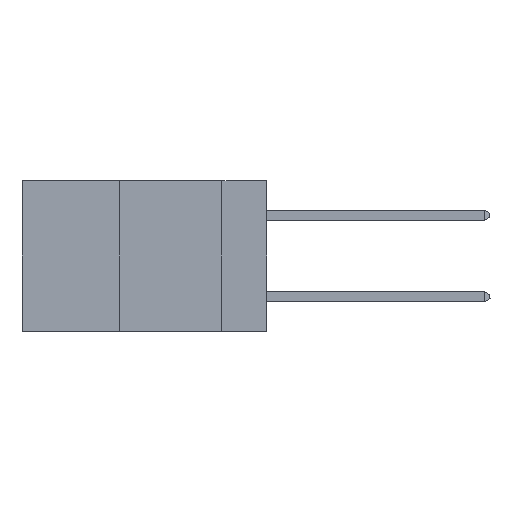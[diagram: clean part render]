
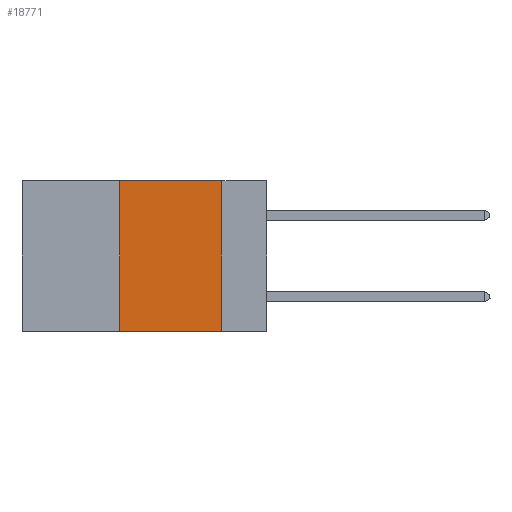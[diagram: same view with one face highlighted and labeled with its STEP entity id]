
A CAD part, left-side view. The second image highlights one B-rep face of the part: STEP entity #18771.
In plain terms, the highlighted planar face has unit normal (-1, 0, 0).
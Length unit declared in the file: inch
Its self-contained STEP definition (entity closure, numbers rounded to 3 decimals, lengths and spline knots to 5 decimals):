
#37 = DIRECTION ( 'NONE',  ( 0., -1., 0. ) ) ;
#182 = EDGE_LOOP ( 'NONE', ( #11099, #10908, #13843, #3437 ) ) ;
#1184 = CARTESIAN_POINT ( 'NONE',  ( 0., 0.11, -0.37 ) ) ;
#2334 = EDGE_CURVE ( 'NONE', #25566, #15913, #15194, .T. ) ;
#3437 = ORIENTED_EDGE ( 'NONE', *, *, #22209, .T. ) ;
#5357 = AXIS2_PLACEMENT_3D ( 'NONE', #20196, #9175, #24572 ) ;
#6641 = DIRECTION ( 'NONE',  ( 0., -1., 0. ) ) ;
#6852 = CARTESIAN_POINT ( 'NONE',  ( 0., 0.36, 0. ) ) ;
#8750 = LINE ( 'NONE', #27980, #25551 ) ;
#9175 = DIRECTION ( 'NONE',  ( 1., 0., 0. ) ) ;
#10634 = DIRECTION ( 'NONE',  ( 0., 0., -1. ) ) ;
#10908 = ORIENTED_EDGE ( 'NONE', *, *, #2334, .F. ) ;
#11099 = ORIENTED_EDGE ( 'NONE', *, *, #18567, .F. ) ;
#12340 = LINE ( 'NONE', #19995, #18293 ) ;
#13843 = ORIENTED_EDGE ( 'NONE', *, *, #27110, .F. ) ;
#14603 = CARTESIAN_POINT ( 'NONE',  ( 0., 0.36, -0.37 ) ) ;
#15194 = LINE ( 'NONE', #27209, #15899 ) ;
#15899 = VECTOR ( 'NONE', #37, 39.37008 ) ;
#15913 = VERTEX_POINT ( 'NONE', #21121 ) ;
#17931 = LINE ( 'NONE', #6852, #26656 ) ;
#18063 = PLANE ( 'NONE',  #5357 ) ;
#18293 = VECTOR ( 'NONE', #6641, 39.37008 ) ;
#18567 = EDGE_CURVE ( 'NONE', #15913, #23486, #8750, .T. ) ;
#18771 = ADVANCED_FACE ( 'NONE', ( #27206 ), #18063, .F. ) ;
#19399 = CARTESIAN_POINT ( 'NONE',  ( 0., 0.36, 0. ) ) ;
#19995 = CARTESIAN_POINT ( 'NONE',  ( 0., 0.6, -0.37 ) ) ;
#20196 = CARTESIAN_POINT ( 'NONE',  ( 0., 0.6, 0. ) ) ;
#21121 = CARTESIAN_POINT ( 'NONE',  ( 0., 0.11, 0. ) ) ;
#22209 = EDGE_CURVE ( 'NONE', #24139, #23486, #12340, .T. ) ;
#22356 = DIRECTION ( 'NONE',  ( 0., 0., 1. ) ) ;
#23486 = VERTEX_POINT ( 'NONE', #1184 ) ;
#24139 = VERTEX_POINT ( 'NONE', #14603 ) ;
#24572 = DIRECTION ( 'NONE',  ( 0., 0., -1. ) ) ;
#25551 = VECTOR ( 'NONE', #10634, 39.37008 ) ;
#25566 = VERTEX_POINT ( 'NONE', #19399 ) ;
#26656 = VECTOR ( 'NONE', #22356, 39.37008 ) ;
#27110 = EDGE_CURVE ( 'NONE', #24139, #25566, #17931, .T. ) ;
#27206 = FACE_OUTER_BOUND ( 'NONE', #182, .T. ) ;
#27209 = CARTESIAN_POINT ( 'NONE',  ( 0., 0.6, 0. ) ) ;
#27980 = CARTESIAN_POINT ( 'NONE',  ( 0., 0.11, 0. ) ) ;
